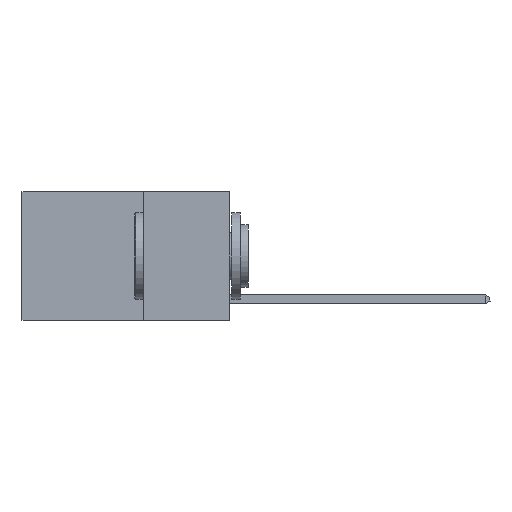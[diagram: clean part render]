
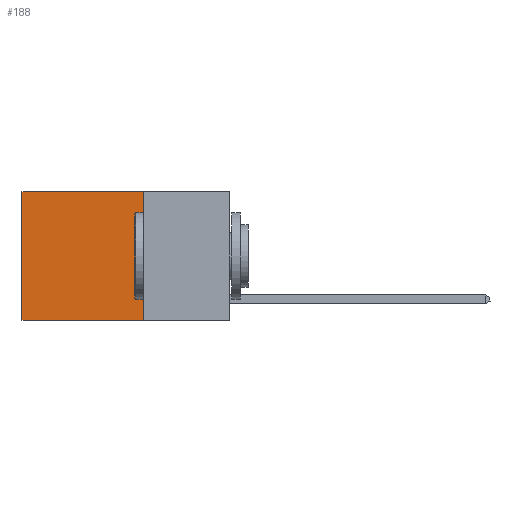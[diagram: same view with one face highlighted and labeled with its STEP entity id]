
A CAD part, left-side view. The second image highlights one B-rep face of the part: STEP entity #188.
In plain terms, the highlighted planar face has unit normal (-1, 0, 0).
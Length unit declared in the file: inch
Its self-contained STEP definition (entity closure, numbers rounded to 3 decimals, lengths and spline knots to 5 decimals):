
#110 = CARTESIAN_POINT ( 'NONE',  ( 0.2625, 0.6, 0. ) ) ;
#188 = ADVANCED_FACE ( 'NONE', ( #6130 ), #3904, .F. ) ;
#783 = CARTESIAN_POINT ( 'NONE',  ( 0.2625, 0.25, 0. ) ) ;
#2297 = DIRECTION ( 'NONE',  ( 0., 0., -1. ) ) ;
#2359 = EDGE_CURVE ( 'NONE', #5235, #3312, #4947, .T. ) ;
#2554 = CARTESIAN_POINT ( 'NONE',  ( 0.2625, 0.6, -0.37 ) ) ;
#3246 = CARTESIAN_POINT ( 'NONE',  ( 0.2625, 0.25, -0.37 ) ) ;
#3253 = CARTESIAN_POINT ( 'NONE',  ( 0.2625, 0.6, 0. ) ) ;
#3312 = VERTEX_POINT ( 'NONE', #110 ) ;
#3501 = VECTOR ( 'NONE', #6200, 39.37008 ) ;
#3773 = CARTESIAN_POINT ( 'NONE',  ( 0.2625, 0.25, 0. ) ) ;
#3904 = PLANE ( 'NONE',  #10972 ) ;
#4022 = VECTOR ( 'NONE', #10959, 39.37008 ) ;
#4875 = EDGE_LOOP ( 'NONE', ( #8941, #9511, #5202, #10226 ) ) ;
#4947 = LINE ( 'NONE', #783, #4022 ) ;
#5202 = ORIENTED_EDGE ( 'NONE', *, *, #5682, .F. ) ;
#5235 = VERTEX_POINT ( 'NONE', #9446 ) ;
#5682 = EDGE_CURVE ( 'NONE', #5235, #6268, #9721, .T. ) ;
#5837 = DIRECTION ( 'NONE',  ( 0., 0., -1. ) ) ;
#5894 = VECTOR ( 'NONE', #7954, 39.37008 ) ;
#6114 = VERTEX_POINT ( 'NONE', #2554 ) ;
#6130 = FACE_OUTER_BOUND ( 'NONE', #4875, .T. ) ;
#6200 = DIRECTION ( 'NONE',  ( 0., 1., 0. ) ) ;
#6268 = VERTEX_POINT ( 'NONE', #3246 ) ;
#7349 = LINE ( 'NONE', #9910, #3501 ) ;
#7648 = EDGE_CURVE ( 'NONE', #6268, #6114, #7349, .T. ) ;
#7754 = DIRECTION ( 'NONE',  ( 1., 0., 0. ) ) ;
#7915 = CARTESIAN_POINT ( 'NONE',  ( 0.2625, 0.25, 0. ) ) ;
#7954 = DIRECTION ( 'NONE',  ( 0., 0., -1. ) ) ;
#8941 = ORIENTED_EDGE ( 'NONE', *, *, #12088, .T. ) ;
#9446 = CARTESIAN_POINT ( 'NONE',  ( 0.2625, 0.25, 0. ) ) ;
#9511 = ORIENTED_EDGE ( 'NONE', *, *, #7648, .F. ) ;
#9721 = LINE ( 'NONE', #7915, #5894 ) ;
#9910 = CARTESIAN_POINT ( 'NONE',  ( 0.2625, 0.25, -0.37 ) ) ;
#10226 = ORIENTED_EDGE ( 'NONE', *, *, #2359, .T. ) ;
#10959 = DIRECTION ( 'NONE',  ( 0., 1., 0. ) ) ;
#10972 = AXIS2_PLACEMENT_3D ( 'NONE', #3773, #7754, #5837 ) ;
#11874 = VECTOR ( 'NONE', #2297, 39.37008 ) ;
#12034 = LINE ( 'NONE', #3253, #11874 ) ;
#12088 = EDGE_CURVE ( 'NONE', #3312, #6114, #12034, .T. ) ;
